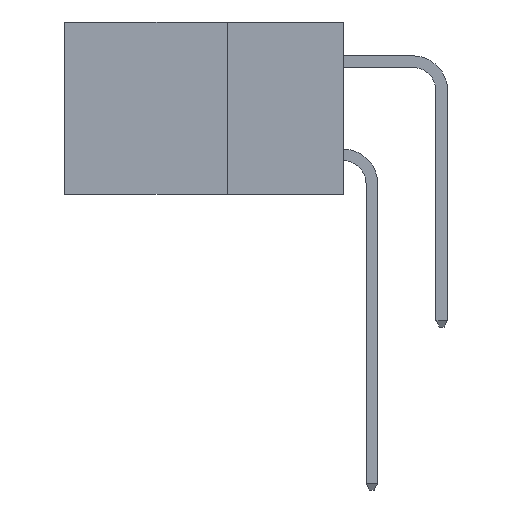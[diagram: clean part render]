
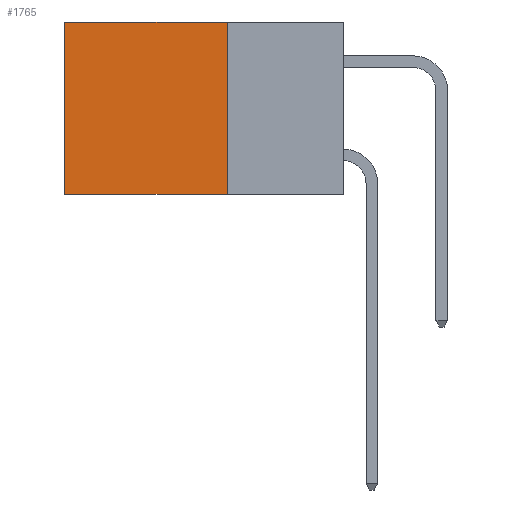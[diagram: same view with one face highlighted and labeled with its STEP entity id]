
A CAD part, left-side view. The second image highlights one B-rep face of the part: STEP entity #1765.
In plain terms, the highlighted planar face has unit normal (-1, 0, 0).
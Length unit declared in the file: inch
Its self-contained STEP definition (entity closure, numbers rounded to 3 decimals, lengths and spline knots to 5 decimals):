
#72 = ORIENTED_EDGE ( 'NONE', *, *, #5644, .T. ) ;
#448 = VERTEX_POINT ( 'NONE', #5922 ) ;
#810 = FACE_OUTER_BOUND ( 'NONE', #4759, .T. ) ;
#1765 = ADVANCED_FACE ( 'NONE', ( #810 ), #12351, .F. ) ;
#1822 = DIRECTION ( 'NONE',  ( 1., 0., 0. ) ) ;
#2011 = VECTOR ( 'NONE', #7343, 39.37008 ) ;
#3243 = VECTOR ( 'NONE', #7220, 39.37008 ) ;
#3568 = DIRECTION ( 'NONE',  ( 0., 0., -1. ) ) ;
#4080 = VECTOR ( 'NONE', #8358, 39.37008 ) ;
#4209 = CARTESIAN_POINT ( 'NONE',  ( 0.2615, 0.6, -0.37 ) ) ;
#4396 = CARTESIAN_POINT ( 'NONE',  ( 0.2615, 0.6, 0. ) ) ;
#4511 = LINE ( 'NONE', #7751, #11789 ) ;
#4759 = EDGE_LOOP ( 'NONE', ( #8540, #6663, #10845, #72 ) ) ;
#5054 = AXIS2_PLACEMENT_3D ( 'NONE', #12236, #1822, #3568 ) ;
#5069 = EDGE_CURVE ( 'NONE', #6084, #448, #8895, .T. ) ;
#5462 = VERTEX_POINT ( 'NONE', #4396 ) ;
#5644 = EDGE_CURVE ( 'NONE', #6084, #5462, #4511, .T. ) ;
#5922 = CARTESIAN_POINT ( 'NONE',  ( 0.2615, 0.25, -0.37 ) ) ;
#6084 = VERTEX_POINT ( 'NONE', #6900 ) ;
#6663 = ORIENTED_EDGE ( 'NONE', *, *, #11751, .F. ) ;
#6900 = CARTESIAN_POINT ( 'NONE',  ( 0.2615, 0.25, 0. ) ) ;
#7220 = DIRECTION ( 'NONE',  ( 0., 1., 0. ) ) ;
#7343 = DIRECTION ( 'NONE',  ( 0., 0., -1. ) ) ;
#7676 = CARTESIAN_POINT ( 'NONE',  ( 0.2615, 0.25, -0.37 ) ) ;
#7718 = VERTEX_POINT ( 'NONE', #4209 ) ;
#7751 = CARTESIAN_POINT ( 'NONE',  ( 0.2615, 0.25, 0. ) ) ;
#7919 = DIRECTION ( 'NONE',  ( 0., 1., 0. ) ) ;
#8358 = DIRECTION ( 'NONE',  ( 0., 0., -1. ) ) ;
#8540 = ORIENTED_EDGE ( 'NONE', *, *, #11868, .T. ) ;
#8895 = LINE ( 'NONE', #7676, #4080 ) ;
#10280 = CARTESIAN_POINT ( 'NONE',  ( 0.2615, 0.6, -0.37 ) ) ;
#10845 = ORIENTED_EDGE ( 'NONE', *, *, #5069, .F. ) ;
#10891 = LINE ( 'NONE', #11951, #3243 ) ;
#11751 = EDGE_CURVE ( 'NONE', #448, #7718, #10891, .T. ) ;
#11789 = VECTOR ( 'NONE', #7919, 39.37008 ) ;
#11868 = EDGE_CURVE ( 'NONE', #5462, #7718, #12154, .T. ) ;
#11951 = CARTESIAN_POINT ( 'NONE',  ( 0.2615, 0.25, -0.37 ) ) ;
#12154 = LINE ( 'NONE', #10280, #2011 ) ;
#12236 = CARTESIAN_POINT ( 'NONE',  ( 0.2615, 0.25, -0.37 ) ) ;
#12351 = PLANE ( 'NONE',  #5054 ) ;
